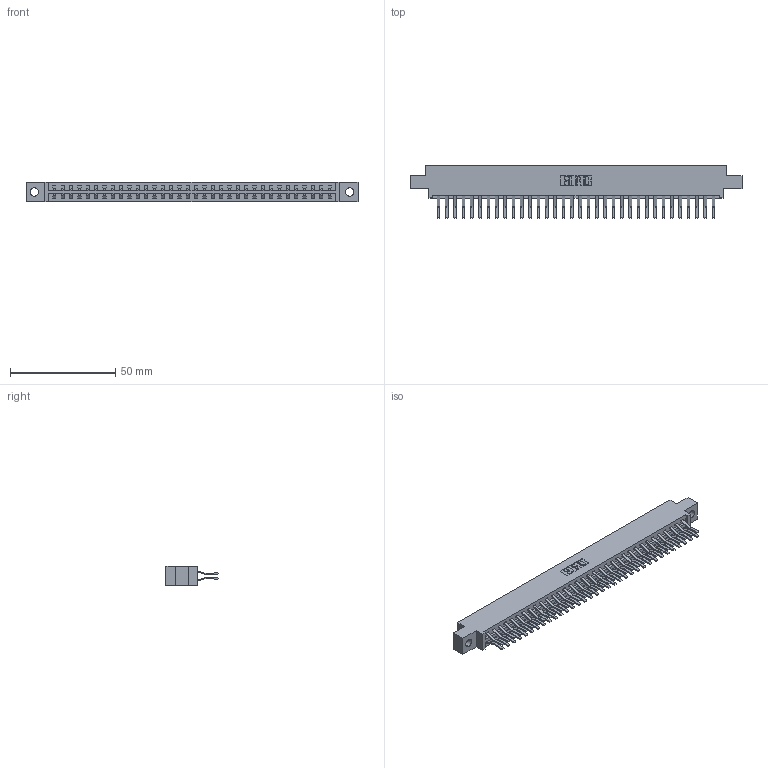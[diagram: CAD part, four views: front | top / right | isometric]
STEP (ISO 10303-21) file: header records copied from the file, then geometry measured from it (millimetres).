
FILE_DESCRIPTION (( 'STEP AP203' ), '1' );
FILE_NAME ('337-068-560-804.STEP', '2019-10-12T02:50:37', ( '' ), ( '' ), 'SwSTEP 2.0', 'SolidWorks 2016', '' );
FILE_SCHEMA (( 'CONFIG_CONTROL_DESIGN' ));
Length unit declared in the file: inch
Products named in the file (3): 345-292-001_560 Tail; 337 Part_0.170 Offset - 0.156 Dia-TH; 337-068-560-804
Assembly tree (69 placements, depth 2):
  337-068-560-804
    337 Part_0.170 Offset - 0.156 Dia-TH
    345-292-001_560 Tail  x68
Bounding box: 157.73 x 24.78 x 9.4 mm (x, y, z)
Volume: 16757.1 mm3; surface area: 20061.5 mm2
Topology: 69 solids, 69 shells, 3926 faces, 11679 edges, 7694 vertices
Faces by surface type: plane 2658, cylinder 1268
Entity records: 27619 total; most frequent: CARTESIAN_POINT 4662, ORIENTED_EDGE 4598, DIRECTION 3983, EDGE_CURVE 2299, LINE 2167, VECTOR 2167, VERTEX_POINT 1530, AXIS2_PLACEMENT_3D 908
